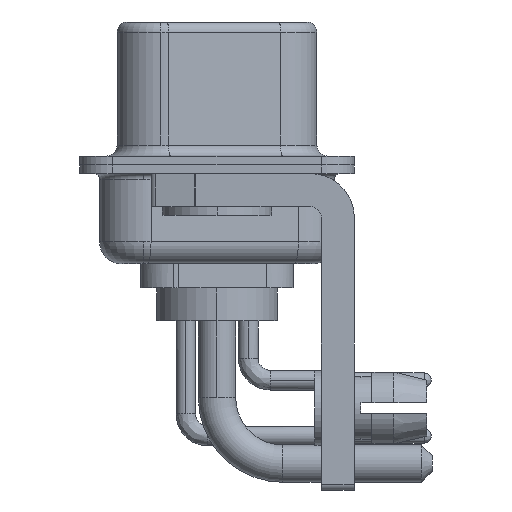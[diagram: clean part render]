
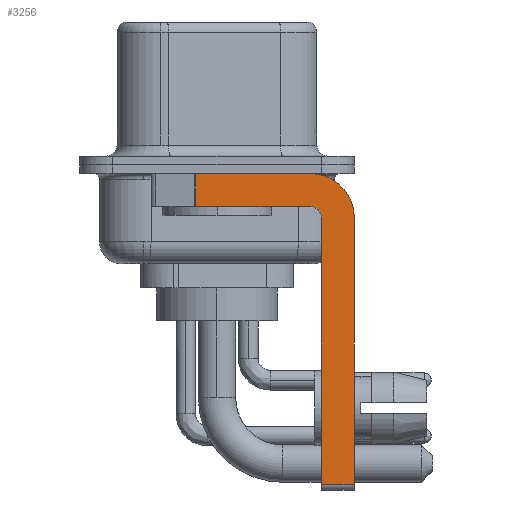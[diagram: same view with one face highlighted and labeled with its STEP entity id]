
A CAD part, left-side view. The second image highlights one B-rep face of the part: STEP entity #3256.
In plain terms, the highlighted planar face has unit normal (-1, 0, 0).
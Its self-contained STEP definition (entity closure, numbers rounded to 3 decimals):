
#491 = ORIENTED_EDGE ( 'NONE', *, *, #603, .F. ) ;
#603 = EDGE_CURVE ( 'NONE', #27751, #11760, #9532, .T. ) ;
#1037 = FACE_OUTER_BOUND ( 'NONE', #1917, .T. ) ;
#1420 = CARTESIAN_POINT ( 'NONE',  ( -2.9, -6.25, -2.4 ) ) ;
#1452 = VECTOR ( 'NONE', #27424, 1000. ) ;
#1491 = CARTESIAN_POINT ( 'NONE',  ( -2.9, -4.25, -2.4 ) ) ;
#1694 = DIRECTION ( 'NONE',  ( 0., -1., 0. ) ) ;
#1917 = EDGE_LOOP ( 'NONE', ( #9597, #28496, #21412, #7799, #16934, #19078, #17398, #491 ) ) ;
#2346 = CARTESIAN_POINT ( 'NONE',  ( -2.9, 0.978, -1.9 ) ) ;
#2679 = VERTEX_POINT ( 'NONE', #9299 ) ;
#2968 = CARTESIAN_POINT ( 'NONE',  ( -2.9, -4.25, -2.4 ) ) ;
#3256 = ADVANCED_FACE ( 'NONE', ( #1037 ), #22992, .F. ) ;
#3423 = AXIS2_PLACEMENT_3D ( 'NONE', #1491, #12928, #10321 ) ;
#3713 = VECTOR ( 'NONE', #25749, 1000. ) ;
#4051 = LINE ( 'NONE', #12866, #8024 ) ;
#4277 = CARTESIAN_POINT ( 'NONE',  ( -2.9, -4.75, -14.8 ) ) ;
#4482 = VERTEX_POINT ( 'NONE', #2346 ) ;
#4565 = CARTESIAN_POINT ( 'NONE',  ( -2.9, 0.978, -1.9 ) ) ;
#4630 = VERTEX_POINT ( 'NONE', #26154 ) ;
#5067 = CIRCLE ( 'NONE', #21991, 0.5 ) ;
#5108 = LINE ( 'NONE', #18636, #9377 ) ;
#5290 = CARTESIAN_POINT ( 'NONE',  ( -2.9, -6.25, -2.4 ) ) ;
#5570 = VECTOR ( 'NONE', #20310, 1000. ) ;
#5625 = DIRECTION ( 'NONE',  ( 0., 0., 1. ) ) ;
#6204 = EDGE_CURVE ( 'NONE', #4630, #27751, #5108, .T. ) ;
#6586 = EDGE_CURVE ( 'NONE', #28971, #17909, #4051, .T. ) ;
#7799 = ORIENTED_EDGE ( 'NONE', *, *, #17810, .F. ) ;
#7959 = DIRECTION ( 'NONE',  ( 1., 0., 0. ) ) ;
#8024 = VECTOR ( 'NONE', #1694, 1000. ) ;
#8501 = VERTEX_POINT ( 'NONE', #18333 ) ;
#9299 = CARTESIAN_POINT ( 'NONE',  ( -2.9, -4.25, -1.9 ) ) ;
#9377 = VECTOR ( 'NONE', #27671, 1000. ) ;
#9532 = CIRCLE ( 'NONE', #3423, 2. ) ;
#9597 = ORIENTED_EDGE ( 'NONE', *, *, #6204, .F. ) ;
#10089 = CARTESIAN_POINT ( 'NONE',  ( -2.9, -4.75, -14.55 ) ) ;
#10321 = DIRECTION ( 'NONE',  ( 0., 0., -1. ) ) ;
#10629 = DIRECTION ( 'NONE',  ( 0., 1., 0. ) ) ;
#11030 = CARTESIAN_POINT ( 'NONE',  ( -2.9, -4.25, -0.4 ) ) ;
#11760 = VERTEX_POINT ( 'NONE', #5290 ) ;
#12866 = CARTESIAN_POINT ( 'NONE',  ( -2.9, -4.25, -14.55 ) ) ;
#12928 = DIRECTION ( 'NONE',  ( 1., 0., 0. ) ) ;
#13516 = LINE ( 'NONE', #4565, #5570 ) ;
#14259 = DIRECTION ( 'NONE',  ( 0., 0., -1. ) ) ;
#16784 = DIRECTION ( 'NONE',  ( -1., 0., 0. ) ) ;
#16934 = ORIENTED_EDGE ( 'NONE', *, *, #27765, .F. ) ;
#17146 = AXIS2_PLACEMENT_3D ( 'NONE', #18831, #7959, #14259 ) ;
#17398 = ORIENTED_EDGE ( 'NONE', *, *, #20351, .F. ) ;
#17810 = EDGE_CURVE ( 'NONE', #8501, #2679, #5067, .T. ) ;
#17909 = VERTEX_POINT ( 'NONE', #28338 ) ;
#18248 = EDGE_CURVE ( 'NONE', #4630, #4482, #13516, .T. ) ;
#18333 = CARTESIAN_POINT ( 'NONE',  ( -2.9, -4.75, -2.4 ) ) ;
#18636 = CARTESIAN_POINT ( 'NONE',  ( -2.9, 3., -0.4 ) ) ;
#18831 = CARTESIAN_POINT ( 'NONE',  ( -2.9, -4.25, -2.4 ) ) ;
#19078 = ORIENTED_EDGE ( 'NONE', *, *, #6586, .T. ) ;
#20310 = DIRECTION ( 'NONE',  ( 0., 0., -1. ) ) ;
#20351 = EDGE_CURVE ( 'NONE', #11760, #17909, #23821, .T. ) ;
#21412 = ORIENTED_EDGE ( 'NONE', *, *, #22650, .F. ) ;
#21991 = AXIS2_PLACEMENT_3D ( 'NONE', #2968, #16784, #5625 ) ;
#22650 = EDGE_CURVE ( 'NONE', #2679, #4482, #27336, .T. ) ;
#22837 = LINE ( 'NONE', #4277, #1452 ) ;
#22992 = PLANE ( 'NONE',  #17146 ) ;
#23821 = LINE ( 'NONE', #1420, #3713 ) ;
#24056 = VECTOR ( 'NONE', #10629, 1000. ) ;
#25134 = CARTESIAN_POINT ( 'NONE',  ( -2.9, -4.25, -1.9 ) ) ;
#25749 = DIRECTION ( 'NONE',  ( 0., 0., -1. ) ) ;
#26154 = CARTESIAN_POINT ( 'NONE',  ( -2.9, 0.978, -0.4 ) ) ;
#27336 = LINE ( 'NONE', #25134, #24056 ) ;
#27424 = DIRECTION ( 'NONE',  ( 0., 0., 1. ) ) ;
#27671 = DIRECTION ( 'NONE',  ( 0., -1., 0. ) ) ;
#27751 = VERTEX_POINT ( 'NONE', #11030 ) ;
#27765 = EDGE_CURVE ( 'NONE', #28971, #8501, #22837, .T. ) ;
#28338 = CARTESIAN_POINT ( 'NONE',  ( -2.9, -6.25, -14.55 ) ) ;
#28496 = ORIENTED_EDGE ( 'NONE', *, *, #18248, .T. ) ;
#28971 = VERTEX_POINT ( 'NONE', #10089 ) ;
